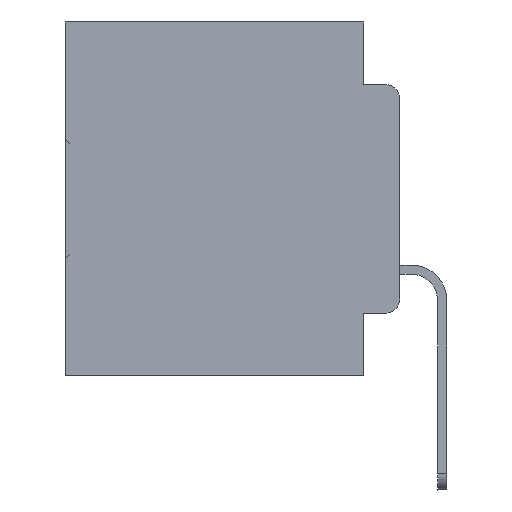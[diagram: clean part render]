
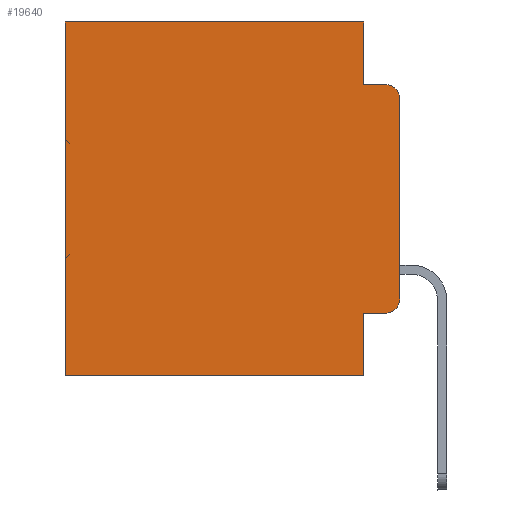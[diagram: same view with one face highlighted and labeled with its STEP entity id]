
A CAD part, left-side view. The second image highlights one B-rep face of the part: STEP entity #19640.
In plain terms, the highlighted planar face has unit normal (-1, 0, 0).
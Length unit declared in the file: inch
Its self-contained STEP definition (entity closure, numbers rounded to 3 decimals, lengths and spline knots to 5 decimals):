
#196 = VECTOR ( 'NONE', #7067, 39.37008 ) ;
#1086 = PLANE ( 'NONE',  #31379 ) ;
#1400 = VERTEX_POINT ( 'NONE', #10291 ) ;
#1833 = ORIENTED_EDGE ( 'NONE', *, *, #4001, .F. ) ;
#1916 = CARTESIAN_POINT ( 'NONE',  ( 0.298, 0.051, -0.4115 ) ) ;
#2300 = DIRECTION ( 'NONE',  ( 0., 0., -1. ) ) ;
#2628 = CARTESIAN_POINT ( 'NONE',  ( 0.298, 0.051, -0.5 ) ) ;
#2715 = CARTESIAN_POINT ( 'NONE',  ( 0.298, 0.051, 0. ) ) ;
#3377 = CARTESIAN_POINT ( 'NONE',  ( 0.298, 0.051, 0. ) ) ;
#3594 = DIRECTION ( 'NONE',  ( 0., 1., 0. ) ) ;
#3762 = LINE ( 'NONE', #27895, #17767 ) ;
#3910 = CARTESIAN_POINT ( 'NONE',  ( 0.298, 0.051, -0.0885 ) ) ;
#4001 = EDGE_CURVE ( 'NONE', #25406, #1400, #15049, .T. ) ;
#4812 = LINE ( 'NONE', #16411, #34075 ) ;
#6316 = VERTEX_POINT ( 'NONE', #2715 ) ;
#6408 = DIRECTION ( 'NONE',  ( 0., 0., -1. ) ) ;
#6450 = CARTESIAN_POINT ( 'NONE',  ( 0.298, 0., 0. ) ) ;
#6794 = CARTESIAN_POINT ( 'NONE',  ( 0.298, 0.051, 0. ) ) ;
#7067 = DIRECTION ( 'NONE',  ( 0., 0., -1. ) ) ;
#7886 = VERTEX_POINT ( 'NONE', #24385 ) ;
#8767 = DIRECTION ( 'NONE',  ( 0., 0., -1. ) ) ;
#9190 = VECTOR ( 'NONE', #20980, 39.37008 ) ;
#9735 = CARTESIAN_POINT ( 'NONE',  ( 0.298, 0.473, 0. ) ) ;
#9886 = ORIENTED_EDGE ( 'NONE', *, *, #35041, .F. ) ;
#10291 = CARTESIAN_POINT ( 'NONE',  ( 0.298, 0.473, -0.5 ) ) ;
#10308 = CARTESIAN_POINT ( 'NONE',  ( 0.298, 0., 0. ) ) ;
#10542 = DIRECTION ( 'NONE',  ( 0., 0., -1. ) ) ;
#11483 = VERTEX_POINT ( 'NONE', #21417 ) ;
#12216 = LINE ( 'NONE', #9735, #196 ) ;
#12942 = CARTESIAN_POINT ( 'NONE',  ( 0.298, 0.051, -0.0885 ) ) ;
#13106 = AXIS2_PLACEMENT_3D ( 'NONE', #27163, #26480, #10542 ) ;
#13253 = ORIENTED_EDGE ( 'NONE', *, *, #23300, .T. ) ;
#14707 = CARTESIAN_POINT ( 'NONE',  ( 0.298, 0.02, -0.4115 ) ) ;
#15049 = LINE ( 'NONE', #31551, #19328 ) ;
#15061 = LINE ( 'NONE', #12942, #29879 ) ;
#15146 = ORIENTED_EDGE ( 'NONE', *, *, #25944, .T. ) ;
#15551 = ORIENTED_EDGE ( 'NONE', *, *, #17411, .F. ) ;
#15774 = DIRECTION ( 'NONE',  ( 0., -1., 0. ) ) ;
#15858 = DIRECTION ( 'NONE',  ( 0., 0., -1. ) ) ;
#15888 = VECTOR ( 'NONE', #6408, 39.37008 ) ;
#16411 = CARTESIAN_POINT ( 'NONE',  ( 0.298, 0.051, -0.4115 ) ) ;
#16843 = LINE ( 'NONE', #3377, #15888 ) ;
#17247 = DIRECTION ( 'NONE',  ( 1., 0., 0. ) ) ;
#17411 = EDGE_CURVE ( 'NONE', #20654, #25406, #16843, .T. ) ;
#17686 = EDGE_CURVE ( 'NONE', #20654, #28171, #4812, .T. ) ;
#17767 = VECTOR ( 'NONE', #3594, 39.37008 ) ;
#19238 = ORIENTED_EDGE ( 'NONE', *, *, #29626, .F. ) ;
#19328 = VECTOR ( 'NONE', #33879, 39.37008 ) ;
#19640 = ADVANCED_FACE ( 'NONE', ( #30746 ), #1086, .F. ) ;
#20654 = VERTEX_POINT ( 'NONE', #1916 ) ;
#20980 = DIRECTION ( 'NONE',  ( 0., 0., -1. ) ) ;
#21215 = DIRECTION ( 'NONE',  ( -1., 0., 0. ) ) ;
#21417 = CARTESIAN_POINT ( 'NONE',  ( 0.298, 0.02, -0.0885 ) ) ;
#22328 = CARTESIAN_POINT ( 'NONE',  ( 0.298, 0., -0.3915 ) ) ;
#23300 = EDGE_CURVE ( 'NONE', #28171, #30948, #33499, .T. ) ;
#23751 = DIRECTION ( 'NONE',  ( 0., -1., 0. ) ) ;
#24131 = ORIENTED_EDGE ( 'NONE', *, *, #29886, .T. ) ;
#24385 = CARTESIAN_POINT ( 'NONE',  ( 0.298, 0., -0.1085 ) ) ;
#24437 = EDGE_CURVE ( 'NONE', #6316, #31535, #31464, .T. ) ;
#25151 = EDGE_LOOP ( 'NONE', ( #19238, #25576, #9886, #25937, #15146, #24131, #1833, #15551, #32071, #13253 ) ) ;
#25406 = VERTEX_POINT ( 'NONE', #2628 ) ;
#25576 = ORIENTED_EDGE ( 'NONE', *, *, #31169, .T. ) ;
#25937 = ORIENTED_EDGE ( 'NONE', *, *, #24437, .F. ) ;
#25944 = EDGE_CURVE ( 'NONE', #6316, #32981, #3762, .T. ) ;
#26480 = DIRECTION ( 'NONE',  ( -1., 0., 0. ) ) ;
#26486 = CARTESIAN_POINT ( 'NONE',  ( 0.298, 0.473, 0. ) ) ;
#27163 = CARTESIAN_POINT ( 'NONE',  ( 0.298, 0.02, -0.3915 ) ) ;
#27895 = CARTESIAN_POINT ( 'NONE',  ( 0.298, 0., 0. ) ) ;
#28171 = VERTEX_POINT ( 'NONE', #14707 ) ;
#29187 = AXIS2_PLACEMENT_3D ( 'NONE', #34713, #21215, #15858 ) ;
#29626 = EDGE_CURVE ( 'NONE', #7886, #30948, #29628, .T. ) ;
#29628 = LINE ( 'NONE', #10308, #29671 ) ;
#29671 = VECTOR ( 'NONE', #2300, 39.37008 ) ;
#29879 = VECTOR ( 'NONE', #23751, 39.37008 ) ;
#29886 = EDGE_CURVE ( 'NONE', #32981, #1400, #12216, .T. ) ;
#30746 = FACE_OUTER_BOUND ( 'NONE', #25151, .T. ) ;
#30948 = VERTEX_POINT ( 'NONE', #22328 ) ;
#31169 = EDGE_CURVE ( 'NONE', #7886, #11483, #31437, .T. ) ;
#31379 = AXIS2_PLACEMENT_3D ( 'NONE', #6450, #17247, #8767 ) ;
#31437 = CIRCLE ( 'NONE', #29187, 0.02 ) ;
#31464 = LINE ( 'NONE', #6794, #9190 ) ;
#31535 = VERTEX_POINT ( 'NONE', #3910 ) ;
#31551 = CARTESIAN_POINT ( 'NONE',  ( 0.298, 0., -0.5 ) ) ;
#32071 = ORIENTED_EDGE ( 'NONE', *, *, #17686, .T. ) ;
#32981 = VERTEX_POINT ( 'NONE', #26486 ) ;
#33499 = CIRCLE ( 'NONE', #13106, 0.02 ) ;
#33879 = DIRECTION ( 'NONE',  ( 0., 1., 0. ) ) ;
#34075 = VECTOR ( 'NONE', #15774, 39.37008 ) ;
#34713 = CARTESIAN_POINT ( 'NONE',  ( 0.298, 0.02, -0.1085 ) ) ;
#35041 = EDGE_CURVE ( 'NONE', #31535, #11483, #15061, .T. ) ;
